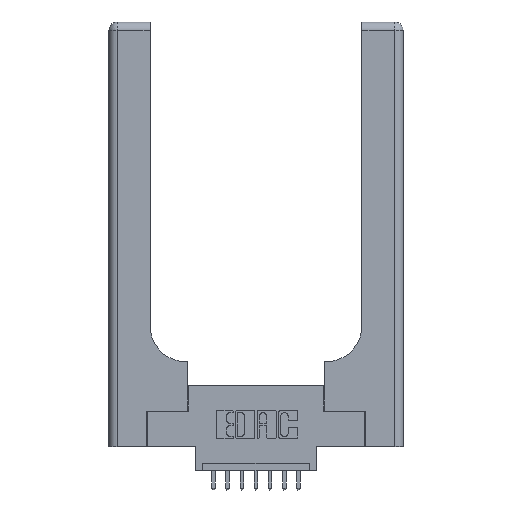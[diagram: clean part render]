
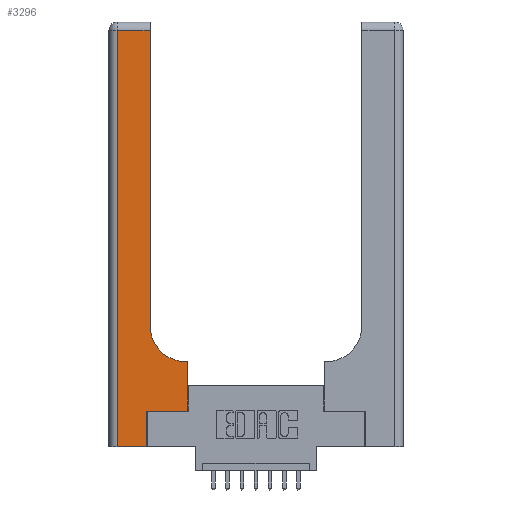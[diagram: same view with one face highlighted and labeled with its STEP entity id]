
A CAD part, top view. The second image highlights one B-rep face of the part: STEP entity #3296.
In plain terms, the highlighted planar face has unit normal (0, 0, 1).
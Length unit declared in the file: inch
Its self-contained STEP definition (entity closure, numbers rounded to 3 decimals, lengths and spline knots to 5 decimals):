
#59 = VECTOR ( 'NONE', #6371, 39.37008 ) ;
#144 = VERTEX_POINT ( 'NONE', #1295 ) ;
#209 = LINE ( 'NONE', #13298, #1650 ) ;
#313 = VERTEX_POINT ( 'NONE', #3911 ) ;
#434 = CIRCLE ( 'NONE', #12535, 0.25 ) ;
#835 = DIRECTION ( 'NONE',  ( 0., 0., -1. ) ) ;
#1023 = ORIENTED_EDGE ( 'NONE', *, *, #12859, .T. ) ;
#1245 = VERTEX_POINT ( 'NONE', #11686 ) ;
#1290 = CARTESIAN_POINT ( 'NONE',  ( 0.269, 0.25, 0.37 ) ) ;
#1295 = CARTESIAN_POINT ( 'NONE',  ( 0.269, 0., 0.37 ) ) ;
#1548 = DIRECTION ( 'NONE',  ( 1., 0., 0. ) ) ;
#1587 = VECTOR ( 'NONE', #12049, 39.37008 ) ;
#1650 = VECTOR ( 'NONE', #9741, 39.37008 ) ;
#1862 = VERTEX_POINT ( 'NONE', #7824 ) ;
#1936 = ORIENTED_EDGE ( 'NONE', *, *, #15195, .T. ) ;
#2140 = LINE ( 'NONE', #7422, #14944 ) ;
#2269 = DIRECTION ( 'NONE',  ( -1., 0., 0. ) ) ;
#2839 = VECTOR ( 'NONE', #10857, 39.37008 ) ;
#3184 = LINE ( 'NONE', #13431, #59 ) ;
#3296 = ADVANCED_FACE ( 'NONE', ( #5142 ), #6922, .F. ) ;
#3655 = CARTESIAN_POINT ( 'NONE',  ( 0.2915, 2.94, 0.37 ) ) ;
#3911 = CARTESIAN_POINT ( 'NONE',  ( 0.06, 2.94, 0.37 ) ) ;
#3924 = CARTESIAN_POINT ( 'NONE',  ( 0., 2.94, 0.37 ) ) ;
#3992 = LINE ( 'NONE', #4991, #1587 ) ;
#4037 = CARTESIAN_POINT ( 'NONE',  ( 0.5415, 0.6, 0.37 ) ) ;
#4248 = CARTESIAN_POINT ( 'NONE',  ( 0.06, 3., 0.37 ) ) ;
#4531 = VECTOR ( 'NONE', #7495, 39.37008 ) ;
#4991 = CARTESIAN_POINT ( 'NONE',  ( 0.5585, 0.25, 0.37 ) ) ;
#5142 = FACE_OUTER_BOUND ( 'NONE', #13630, .T. ) ;
#5943 = CARTESIAN_POINT ( 'NONE',  ( 0., 3., 0.37 ) ) ;
#6371 = DIRECTION ( 'NONE',  ( 0., 1., 0. ) ) ;
#6611 = EDGE_CURVE ( 'NONE', #8074, #12363, #3184, .T. ) ;
#6847 = DIRECTION ( 'NONE',  ( 1., 0., 0. ) ) ;
#6897 = ORIENTED_EDGE ( 'NONE', *, *, #14351, .T. ) ;
#6922 = PLANE ( 'NONE',  #11306 ) ;
#7003 = LINE ( 'NONE', #12039, #8108 ) ;
#7143 = ORIENTED_EDGE ( 'NONE', *, *, #10669, .T. ) ;
#7422 = CARTESIAN_POINT ( 'NONE',  ( 0.269, 0.25, 0.37 ) ) ;
#7495 = DIRECTION ( 'NONE',  ( 0., 1., 0. ) ) ;
#7514 = ORIENTED_EDGE ( 'NONE', *, *, #13386, .T. ) ;
#7824 = CARTESIAN_POINT ( 'NONE',  ( 0.5585, 0.25, 0.37 ) ) ;
#8034 = ORIENTED_EDGE ( 'NONE', *, *, #6611, .T. ) ;
#8074 = VERTEX_POINT ( 'NONE', #8128 ) ;
#8108 = VECTOR ( 'NONE', #10917, 39.37008 ) ;
#8128 = CARTESIAN_POINT ( 'NONE',  ( 0.2915, 0.85, 0.37 ) ) ;
#8207 = DIRECTION ( 'NONE',  ( 0., 0., -1. ) ) ;
#9741 = DIRECTION ( 'NONE',  ( -1., 0., 0. ) ) ;
#9757 = VECTOR ( 'NONE', #13622, 39.37008 ) ;
#10137 = LINE ( 'NONE', #4248, #9757 ) ;
#10427 = CARTESIAN_POINT ( 'NONE',  ( 0.5585, 0.6, 0.37 ) ) ;
#10669 = EDGE_CURVE ( 'NONE', #15255, #14536, #209, .T. ) ;
#10857 = DIRECTION ( 'NONE',  ( -1., 0., 0. ) ) ;
#10917 = DIRECTION ( 'NONE',  ( 1., 0., 0. ) ) ;
#10971 = ORIENTED_EDGE ( 'NONE', *, *, #12099, .T. ) ;
#11209 = EDGE_CURVE ( 'NONE', #1245, #144, #7003, .T. ) ;
#11306 = AXIS2_PLACEMENT_3D ( 'NONE', #5943, #8207, #2269 ) ;
#11686 = CARTESIAN_POINT ( 'NONE',  ( 0.06, 0., 0.37 ) ) ;
#11951 = LINE ( 'NONE', #12336, #4531 ) ;
#11961 = ORIENTED_EDGE ( 'NONE', *, *, #13856, .T. ) ;
#12039 = CARTESIAN_POINT ( 'NONE',  ( 0., 0., 0.37 ) ) ;
#12049 = DIRECTION ( 'NONE',  ( 0., 1., 0. ) ) ;
#12099 = EDGE_CURVE ( 'NONE', #313, #1245, #10137, .T. ) ;
#12336 = CARTESIAN_POINT ( 'NONE',  ( 0.269, 0., 0.37 ) ) ;
#12363 = VERTEX_POINT ( 'NONE', #3655 ) ;
#12480 = ORIENTED_EDGE ( 'NONE', *, *, #11209, .T. ) ;
#12535 = AXIS2_PLACEMENT_3D ( 'NONE', #15001, #835, #6847 ) ;
#12859 = EDGE_CURVE ( 'NONE', #14791, #1862, #2140, .T. ) ;
#13298 = CARTESIAN_POINT ( 'NONE',  ( 0.2915, 0.6, 0.37 ) ) ;
#13386 = EDGE_CURVE ( 'NONE', #1862, #15255, #3992, .T. ) ;
#13431 = CARTESIAN_POINT ( 'NONE',  ( 0.2915, 3., 0.37 ) ) ;
#13622 = DIRECTION ( 'NONE',  ( 0., -1., 0. ) ) ;
#13630 = EDGE_LOOP ( 'NONE', ( #8034, #6897, #10971, #12480, #11961, #1023, #7514, #7143, #1936 ) ) ;
#13856 = EDGE_CURVE ( 'NONE', #144, #14791, #11951, .T. ) ;
#13982 = LINE ( 'NONE', #3924, #2839 ) ;
#14351 = EDGE_CURVE ( 'NONE', #12363, #313, #13982, .T. ) ;
#14536 = VERTEX_POINT ( 'NONE', #4037 ) ;
#14791 = VERTEX_POINT ( 'NONE', #1290 ) ;
#14944 = VECTOR ( 'NONE', #1548, 39.37008 ) ;
#15001 = CARTESIAN_POINT ( 'NONE',  ( 0.5415, 0.85, 0.37 ) ) ;
#15195 = EDGE_CURVE ( 'NONE', #14536, #8074, #434, .T. ) ;
#15255 = VERTEX_POINT ( 'NONE', #10427 ) ;
